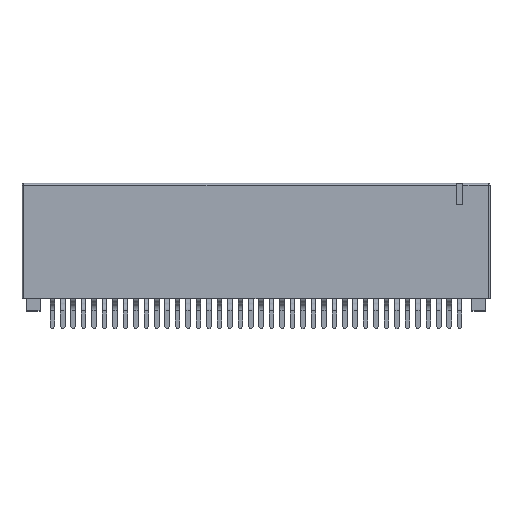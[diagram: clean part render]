
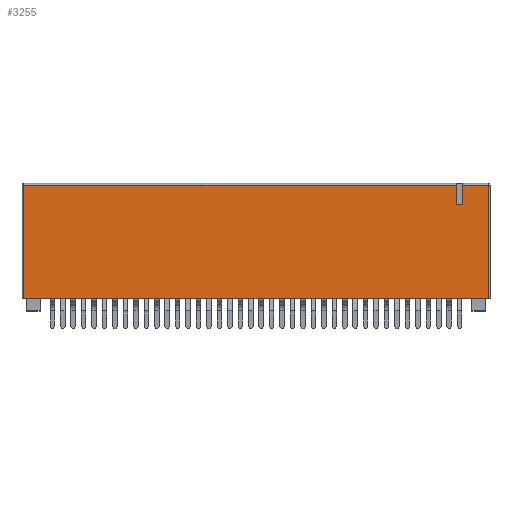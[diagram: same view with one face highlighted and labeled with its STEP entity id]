
A CAD part, top view. The second image highlights one B-rep face of the part: STEP entity #3255.
In plain terms, the highlighted planar face has unit normal (0, 0, 1).
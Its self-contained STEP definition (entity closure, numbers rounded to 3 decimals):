
#527 = EDGE_CURVE ( 'NONE', #15141, #15828, #9628, .T. ) ;
#850 = AXIS2_PLACEMENT_3D ( 'NONE', #22008, #2357, #22158 ) ;
#1537 = VERTEX_POINT ( 'NONE', #5611 ) ;
#1964 = ORIENTED_EDGE ( 'NONE', *, *, #22912, .T. ) ;
#2356 = VERTEX_POINT ( 'NONE', #28268 ) ;
#2357 = DIRECTION ( 'NONE',  ( 0., 0., -1. ) ) ;
#2532 = DIRECTION ( 'NONE',  ( 1., 0., 0. ) ) ;
#2878 = CARTESIAN_POINT ( 'NONE',  ( 56.9, 1.5, 0. ) ) ;
#3255 = ADVANCED_FACE ( 'NONE', ( #25112 ), #30024, .F. ) ;
#3656 = DIRECTION ( 'NONE',  ( -1., 0., 0. ) ) ;
#4539 = CARTESIAN_POINT ( 'NONE',  ( 0.2, 15.5, 0. ) ) ;
#5611 = CARTESIAN_POINT ( 'NONE',  ( 56.7, 1.5, 0. ) ) ;
#5958 = EDGE_CURVE ( 'NONE', #24221, #15141, #30044, .T. ) ;
#6113 = CARTESIAN_POINT ( 'NONE',  ( 0., 15.3, 0. ) ) ;
#7465 = LINE ( 'NONE', #4539, #24755 ) ;
#7497 = LINE ( 'NONE', #19942, #16026 ) ;
#7560 = EDGE_CURVE ( 'NONE', #1537, #2356, #7497, .T. ) ;
#9173 = CARTESIAN_POINT ( 'NONE',  ( 0.2, 1.5, 0. ) ) ;
#9628 = LINE ( 'NONE', #19622, #29842 ) ;
#10201 = ORIENTED_EDGE ( 'NONE', *, *, #23744, .T. ) ;
#10374 = CARTESIAN_POINT ( 'NONE',  ( 52.825, 12.95, 0. ) ) ;
#10475 = VERTEX_POINT ( 'NONE', #9173 ) ;
#11561 = CARTESIAN_POINT ( 'NONE',  ( 53.605, 15.3, 0. ) ) ;
#11670 = VECTOR ( 'NONE', #15159, 1000. ) ;
#11960 = CARTESIAN_POINT ( 'NONE',  ( 52.825, 15.3, 0. ) ) ;
#11994 = LINE ( 'NONE', #26902, #25313 ) ;
#12678 = ORIENTED_EDGE ( 'NONE', *, *, #23114, .F. ) ;
#12774 = EDGE_LOOP ( 'NONE', ( #15147, #17651, #21043, #1964, #12678, #15752, #10201, #29358 ) ) ;
#13723 = CARTESIAN_POINT ( 'NONE',  ( 52.825, 12.95, 0. ) ) ;
#15141 = VERTEX_POINT ( 'NONE', #22429 ) ;
#15147 = ORIENTED_EDGE ( 'NONE', *, *, #5958, .F. ) ;
#15159 = DIRECTION ( 'NONE',  ( -1., 0., 0. ) ) ;
#15752 = ORIENTED_EDGE ( 'NONE', *, *, #7560, .T. ) ;
#15828 = VERTEX_POINT ( 'NONE', #11561 ) ;
#15885 = VECTOR ( 'NONE', #2532, 1000. ) ;
#16026 = VECTOR ( 'NONE', #20441, 1000. ) ;
#16942 = VECTOR ( 'NONE', #23566, 1000. ) ;
#17651 = ORIENTED_EDGE ( 'NONE', *, *, #23891, .T. ) ;
#19478 = EDGE_CURVE ( 'NONE', #31321, #31527, #25934, .T. ) ;
#19622 = CARTESIAN_POINT ( 'NONE',  ( 53.605, 12.95, 0. ) ) ;
#19681 = DIRECTION ( 'NONE',  ( -1., 0., 0. ) ) ;
#19942 = CARTESIAN_POINT ( 'NONE',  ( 56.7, 15.5, 0. ) ) ;
#20441 = DIRECTION ( 'NONE',  ( 0., 1., 0. ) ) ;
#21043 = ORIENTED_EDGE ( 'NONE', *, *, #19478, .T. ) ;
#21228 = VECTOR ( 'NONE', #3656, 1000. ) ;
#22008 = CARTESIAN_POINT ( 'NONE',  ( 0., 15.5, 0. ) ) ;
#22158 = DIRECTION ( 'NONE',  ( -1., 0., 0. ) ) ;
#22429 = CARTESIAN_POINT ( 'NONE',  ( 53.605, 12.95, 0. ) ) ;
#22912 = EDGE_CURVE ( 'NONE', #31527, #10475, #7465, .T. ) ;
#23114 = EDGE_CURVE ( 'NONE', #1537, #10475, #27626, .T. ) ;
#23566 = DIRECTION ( 'NONE',  ( 0., 1., 0. ) ) ;
#23744 = EDGE_CURVE ( 'NONE', #2356, #15828, #11994, .T. ) ;
#23891 = EDGE_CURVE ( 'NONE', #24221, #31321, #31273, .T. ) ;
#24221 = VERTEX_POINT ( 'NONE', #30009 ) ;
#24755 = VECTOR ( 'NONE', #29770, 1000. ) ;
#25112 = FACE_OUTER_BOUND ( 'NONE', #12774, .T. ) ;
#25313 = VECTOR ( 'NONE', #19681, 1000. ) ;
#25698 = CARTESIAN_POINT ( 'NONE',  ( 0.2, 15.3, 0. ) ) ;
#25934 = LINE ( 'NONE', #6113, #21228 ) ;
#26902 = CARTESIAN_POINT ( 'NONE',  ( 0., 15.3, 0. ) ) ;
#27011 = DIRECTION ( 'NONE',  ( 0., 1., 0. ) ) ;
#27626 = LINE ( 'NONE', #2878, #11670 ) ;
#28268 = CARTESIAN_POINT ( 'NONE',  ( 56.7, 15.3, 0. ) ) ;
#29358 = ORIENTED_EDGE ( 'NONE', *, *, #527, .F. ) ;
#29770 = DIRECTION ( 'NONE',  ( 0., -1., 0. ) ) ;
#29842 = VECTOR ( 'NONE', #27011, 1000. ) ;
#30009 = CARTESIAN_POINT ( 'NONE',  ( 52.825, 12.95, 0. ) ) ;
#30024 = PLANE ( 'NONE',  #850 ) ;
#30044 = LINE ( 'NONE', #10374, #15885 ) ;
#31273 = LINE ( 'NONE', #13723, #16942 ) ;
#31321 = VERTEX_POINT ( 'NONE', #11960 ) ;
#31527 = VERTEX_POINT ( 'NONE', #25698 ) ;
